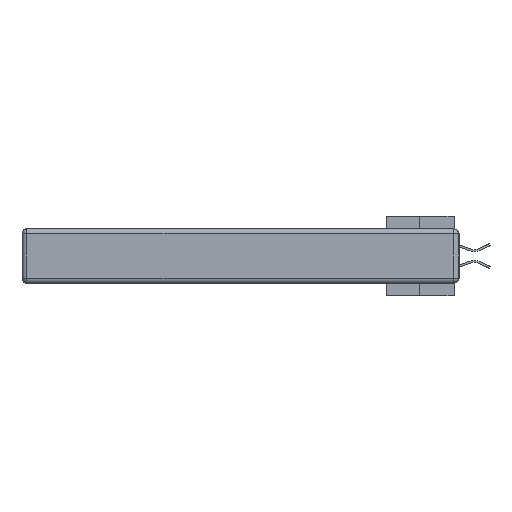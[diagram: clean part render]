
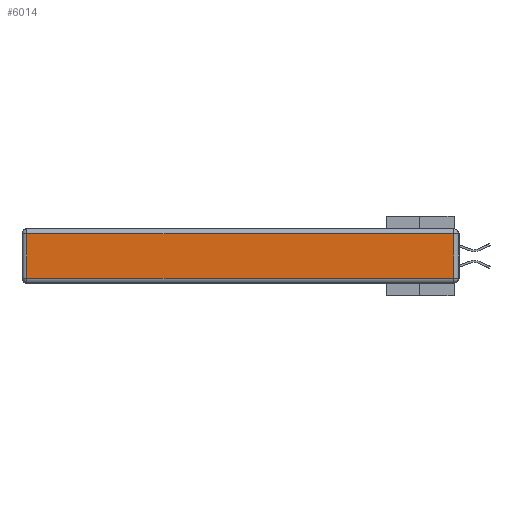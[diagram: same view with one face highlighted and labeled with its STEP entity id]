
A CAD part, left-side view. The second image highlights one B-rep face of the part: STEP entity #6014.
In plain terms, the highlighted planar face has unit normal (-1, 0, 0).
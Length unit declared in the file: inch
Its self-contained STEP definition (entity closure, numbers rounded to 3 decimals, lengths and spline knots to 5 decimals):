
#1268 = VERTEX_POINT ( 'NONE', #29514 ) ;
#2046 = VERTEX_POINT ( 'NONE', #11696 ) ;
#2808 = ORIENTED_EDGE ( 'NONE', *, *, #12925, .T. ) ;
#3587 = AXIS2_PLACEMENT_3D ( 'NONE', #29276, #11187, #5633 ) ;
#4887 = DIRECTION ( 'NONE',  ( 0., -1., 0. ) ) ;
#5633 = DIRECTION ( 'NONE',  ( 0., 0., 1. ) ) ;
#6014 = ADVANCED_FACE ( 'NONE', ( #38684 ), #26128, .T. ) ;
#8834 = EDGE_CURVE ( 'NONE', #2046, #13403, #14170, .T. ) ;
#8981 = VECTOR ( 'NONE', #24369, 39.37008 ) ;
#9021 = VECTOR ( 'NONE', #19265, 39.37008 ) ;
#9186 = VECTOR ( 'NONE', #34225, 39.37008 ) ;
#9766 = ORIENTED_EDGE ( 'NONE', *, *, #13090, .T. ) ;
#11058 = VECTOR ( 'NONE', #4887, 39.37008 ) ;
#11187 = DIRECTION ( 'NONE',  ( -1., 0., 0. ) ) ;
#11349 = CARTESIAN_POINT ( 'NONE',  ( 0., 0., -0.313 ) ) ;
#11696 = CARTESIAN_POINT ( 'NONE',  ( 0., 0.03, -0.03 ) ) ;
#12445 = ORIENTED_EDGE ( 'NONE', *, *, #20077, .T. ) ;
#12925 = EDGE_CURVE ( 'NONE', #1268, #2046, #15789, .T. ) ;
#13090 = EDGE_CURVE ( 'NONE', #35351, #1268, #35980, .T. ) ;
#13403 = VERTEX_POINT ( 'NONE', #30476 ) ;
#14170 = LINE ( 'NONE', #25154, #9021 ) ;
#14496 = ORIENTED_EDGE ( 'NONE', *, *, #8834, .T. ) ;
#15789 = LINE ( 'NONE', #25508, #9186 ) ;
#19265 = DIRECTION ( 'NONE',  ( 0., 1., 0. ) ) ;
#20077 = EDGE_CURVE ( 'NONE', #13403, #35351, #32915, .T. ) ;
#24369 = DIRECTION ( 'NONE',  ( 0., 0., -1. ) ) ;
#25154 = CARTESIAN_POINT ( 'NONE',  ( 0., 2.75, -0.03 ) ) ;
#25508 = CARTESIAN_POINT ( 'NONE',  ( 0., 0.03, -0.343 ) ) ;
#26128 = PLANE ( 'NONE',  #3587 ) ;
#27320 = EDGE_LOOP ( 'NONE', ( #9766, #2808, #14496, #12445 ) ) ;
#29276 = CARTESIAN_POINT ( 'NONE',  ( 0., 0., -0.343 ) ) ;
#29514 = CARTESIAN_POINT ( 'NONE',  ( 0., 0.03, -0.313 ) ) ;
#30298 = CARTESIAN_POINT ( 'NONE',  ( 0., 2.72, -0.343 ) ) ;
#30476 = CARTESIAN_POINT ( 'NONE',  ( 0., 2.72, -0.03 ) ) ;
#32915 = LINE ( 'NONE', #30298, #8981 ) ;
#34225 = DIRECTION ( 'NONE',  ( 0., 0., 1. ) ) ;
#35351 = VERTEX_POINT ( 'NONE', #35493 ) ;
#35493 = CARTESIAN_POINT ( 'NONE',  ( 0., 2.72, -0.313 ) ) ;
#35980 = LINE ( 'NONE', #11349, #11058 ) ;
#38684 = FACE_OUTER_BOUND ( 'NONE', #27320, .T. ) ;
